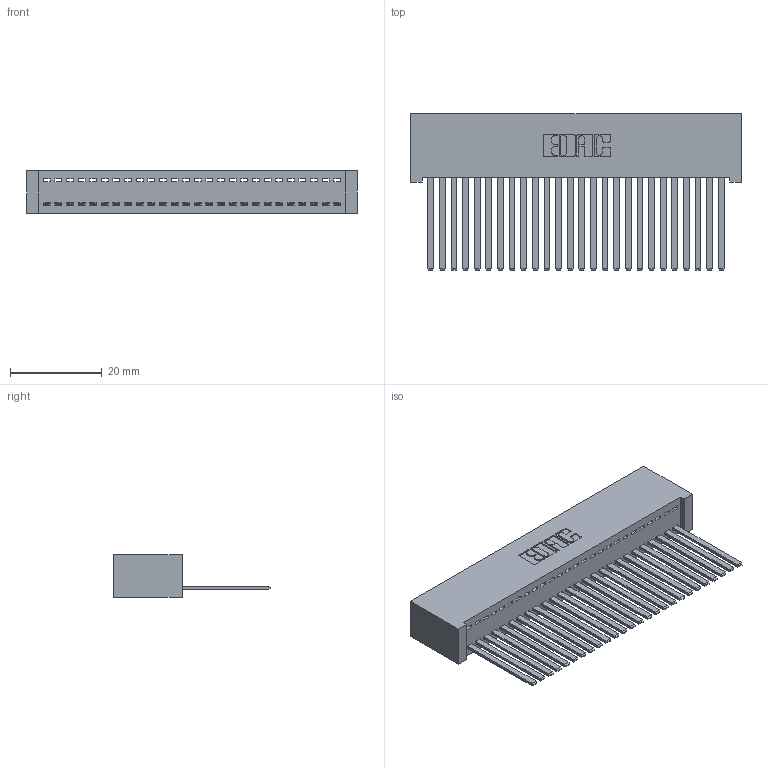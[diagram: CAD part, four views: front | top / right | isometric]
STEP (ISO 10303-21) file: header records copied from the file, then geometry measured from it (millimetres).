
FILE_DESCRIPTION (( 'STEP AP203' ), '1' );
FILE_NAME ('392-026-544-101.STEP', '2018-08-15T15:40:27', ( '' ), ( '' ), 'SwSTEP 2.0', 'SolidWorks 2016', '' );
FILE_SCHEMA (( 'CONFIG_CONTROL_DESIGN' ));
Length unit declared in the file: inch
Products named in the file (3): 342 Part_Lugless; 345-292-001_345-293-144; 392-026-544-101
Assembly tree (27 placements, depth 2):
  392-026-544-101
    342 Part_Lugless
    345-292-001_345-293-144  x26
Bounding box: 72.29 x 34.3 x 9.4 mm (x, y, z)
Volume: 6989.4 mm3; surface area: 11145.2 mm2
Topology: 27 solids, 27 shells, 1454 faces, 4383 edges, 2886 vertices
Faces by surface type: plane 1050, cylinder 404
Entity records: 17371 total; most frequent: CARTESIAN_POINT 3004, ORIENTED_EDGE 2966, DIRECTION 2555, EDGE_CURVE 1483, VECTOR 1367, LINE 1367, VERTEX_POINT 986, AXIS2_PLACEMENT_3D 594
